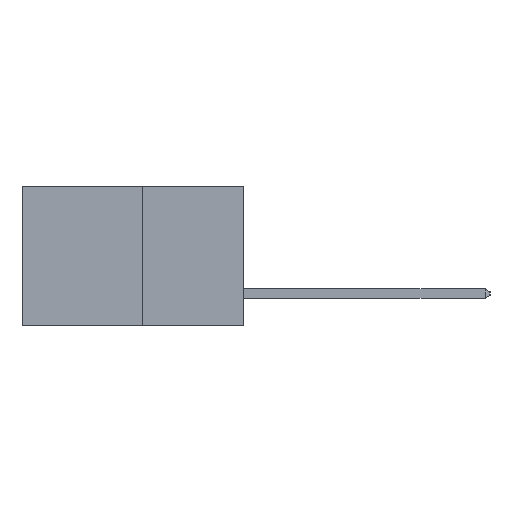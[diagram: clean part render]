
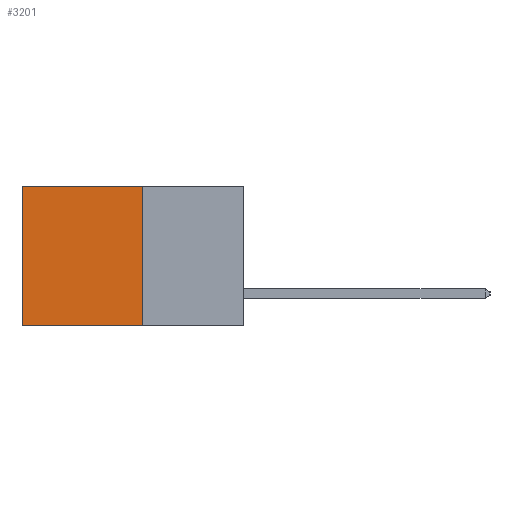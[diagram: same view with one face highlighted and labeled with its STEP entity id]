
A CAD part, left-side view. The second image highlights one B-rep face of the part: STEP entity #3201.
In plain terms, the highlighted planar face has unit normal (-1, 0, 0).
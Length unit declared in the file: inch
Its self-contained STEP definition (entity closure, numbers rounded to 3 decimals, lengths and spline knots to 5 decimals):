
#622 = CARTESIAN_POINT ( 'NONE',  ( 0.277, 0.27, -0.37 ) ) ;
#626 = PLANE ( 'NONE',  #4426 ) ;
#1752 = DIRECTION ( 'NONE',  ( 0., 1., 0. ) ) ;
#1785 = CARTESIAN_POINT ( 'NONE',  ( 0.277, 0.59, -0.37 ) ) ;
#2413 = LINE ( 'NONE', #11889, #12967 ) ;
#3201 = ADVANCED_FACE ( 'NONE', ( #13084 ), #626, .F. ) ;
#3315 = DIRECTION ( 'NONE',  ( 0., 0., -1. ) ) ;
#3944 = VERTEX_POINT ( 'NONE', #4886 ) ;
#4426 = AXIS2_PLACEMENT_3D ( 'NONE', #622, #17859, #17807 ) ;
#4486 = CARTESIAN_POINT ( 'NONE',  ( 0.277, 0.27, 0. ) ) ;
#4582 = VECTOR ( 'NONE', #12257, 39.37008 ) ;
#4886 = CARTESIAN_POINT ( 'NONE',  ( 0.277, 0.59, -0.37 ) ) ;
#5063 = LINE ( 'NONE', #10904, #4582 ) ;
#7661 = EDGE_CURVE ( 'NONE', #17354, #3944, #7822, .T. ) ;
#7822 = LINE ( 'NONE', #1785, #14772 ) ;
#8392 = EDGE_CURVE ( 'NONE', #17969, #13513, #5063, .T. ) ;
#9020 = CARTESIAN_POINT ( 'NONE',  ( 0.277, 0.59, 0. ) ) ;
#10354 = ORIENTED_EDGE ( 'NONE', *, *, #8392, .F. ) ;
#10904 = CARTESIAN_POINT ( 'NONE',  ( 0.277, 0.27, -0.37 ) ) ;
#11889 = CARTESIAN_POINT ( 'NONE',  ( 0.277, 0.27, 0. ) ) ;
#11910 = EDGE_LOOP ( 'NONE', ( #15905, #13553, #10354, #14407 ) ) ;
#12155 = DIRECTION ( 'NONE',  ( 0., 1., 0. ) ) ;
#12257 = DIRECTION ( 'NONE',  ( 0., 0., -1. ) ) ;
#12967 = VECTOR ( 'NONE', #1752, 39.37008 ) ;
#13084 = FACE_OUTER_BOUND ( 'NONE', #11910, .T. ) ;
#13355 = VECTOR ( 'NONE', #12155, 39.37008 ) ;
#13513 = VERTEX_POINT ( 'NONE', #15536 ) ;
#13553 = ORIENTED_EDGE ( 'NONE', *, *, #16195, .F. ) ;
#14407 = ORIENTED_EDGE ( 'NONE', *, *, #17405, .T. ) ;
#14772 = VECTOR ( 'NONE', #3315, 39.37008 ) ;
#15536 = CARTESIAN_POINT ( 'NONE',  ( 0.277, 0.27, -0.37 ) ) ;
#15905 = ORIENTED_EDGE ( 'NONE', *, *, #7661, .T. ) ;
#16195 = EDGE_CURVE ( 'NONE', #13513, #3944, #17332, .T. ) ;
#17332 = LINE ( 'NONE', #17551, #13355 ) ;
#17354 = VERTEX_POINT ( 'NONE', #9020 ) ;
#17405 = EDGE_CURVE ( 'NONE', #17969, #17354, #2413, .T. ) ;
#17551 = CARTESIAN_POINT ( 'NONE',  ( 0.277, 0.27, -0.37 ) ) ;
#17807 = DIRECTION ( 'NONE',  ( 0., 0., -1. ) ) ;
#17859 = DIRECTION ( 'NONE',  ( 1., 0., 0. ) ) ;
#17969 = VERTEX_POINT ( 'NONE', #4486 ) ;
